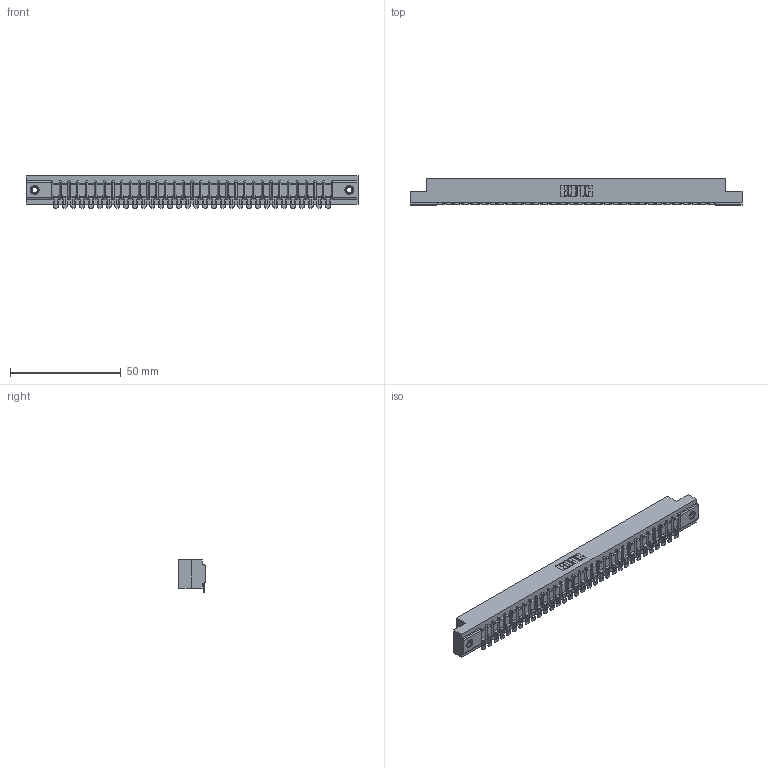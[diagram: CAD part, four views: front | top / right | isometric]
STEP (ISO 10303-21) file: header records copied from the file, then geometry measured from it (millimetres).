
FILE_DESCRIPTION (( 'STEP AP203' ), '1' );
FILE_NAME ('357-032-554-107.STEP', '2019-09-17T04:27:57', ( '' ), ( '' ), 'SwSTEP 2.0', 'SolidWorks 2016', '' );
FILE_SCHEMA (( 'CONFIG_CONTROL_DESIGN' ));
Length unit declared in the file: inch
Products named in the file (4): 307 Part_.156 Dia Mounting Holes; 357-032-554-107; 307-290-002_554; 345-250-001_345-250-005-103
Assembly tree (35 placements, depth 2):
  357-032-554-107
    307 Part_.156 Dia Mounting Holes
    307-290-002_554  x32
    345-250-001_345-250-005-103  x2
Bounding box: 149.81 x 12.01 x 14.52 mm (x, y, z)
Volume: 15954.9 mm3; surface area: 19997.9 mm2
Topology: 35 solids, 35 shells, 2803 faces, 8555 edges, 5606 vertices
Faces by surface type: plane 1574, cylinder 1147, sphere 66, cone 12, torus 4
Entity records: 30816 total; most frequent: CARTESIAN_POINT 5177, ORIENTED_EDGE 5160, DIRECTION 5050, EDGE_CURVE 2580, VECTOR 1964, LINE 1964, VERTEX_POINT 1670, AXIS2_PLACEMENT_3D 1543
